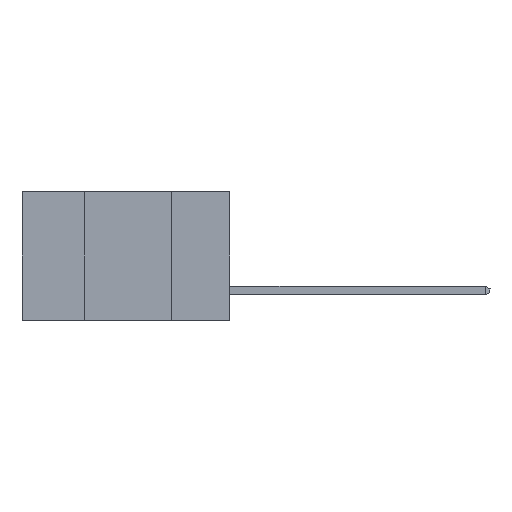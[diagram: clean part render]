
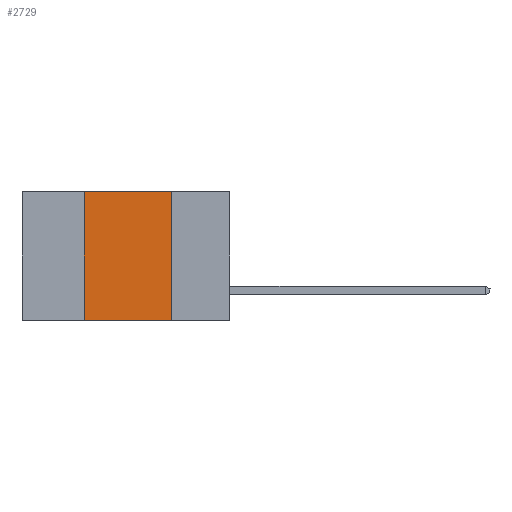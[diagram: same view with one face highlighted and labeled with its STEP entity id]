
A CAD part, left-side view. The second image highlights one B-rep face of the part: STEP entity #2729.
In plain terms, the highlighted planar face has unit normal (-1, 0, 0).
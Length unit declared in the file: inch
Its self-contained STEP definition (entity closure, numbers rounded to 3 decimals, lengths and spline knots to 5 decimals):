
#408 = ORIENTED_EDGE ( 'NONE', *, *, #13602, .F. ) ;
#1017 = EDGE_CURVE ( 'NONE', #12501, #17342, #10388, .T. ) ;
#1436 = VERTEX_POINT ( 'NONE', #19409 ) ;
#1492 = DIRECTION ( 'NONE',  ( 0., -1., 0. ) ) ;
#1813 = LINE ( 'NONE', #13632, #11678 ) ;
#1953 = CARTESIAN_POINT ( 'NONE',  ( 0., 0.17, -0.37 ) ) ;
#2729 = ADVANCED_FACE ( 'NONE', ( #10214 ), #8572, .F. ) ;
#2886 = DIRECTION ( 'NONE',  ( 0., 0., -1. ) ) ;
#4123 = AXIS2_PLACEMENT_3D ( 'NONE', #11872, #16969, #15203 ) ;
#4534 = CARTESIAN_POINT ( 'NONE',  ( 0., 0.17, -0.37 ) ) ;
#5583 = ORIENTED_EDGE ( 'NONE', *, *, #14785, .T. ) ;
#5584 = VERTEX_POINT ( 'NONE', #8233 ) ;
#6605 = LINE ( 'NONE', #11573, #21683 ) ;
#7022 = DIRECTION ( 'NONE',  ( 0., 0., 1. ) ) ;
#8233 = CARTESIAN_POINT ( 'NONE',  ( 0., 0.42, -0.37 ) ) ;
#8572 = PLANE ( 'NONE',  #4123 ) ;
#10214 = FACE_OUTER_BOUND ( 'NONE', #13310, .T. ) ;
#10388 = LINE ( 'NONE', #4534, #18707 ) ;
#10633 = ORIENTED_EDGE ( 'NONE', *, *, #1017, .F. ) ;
#11573 = CARTESIAN_POINT ( 'NONE',  ( 0., 0.6, 0. ) ) ;
#11678 = VECTOR ( 'NONE', #1492, 39.37008 ) ;
#11872 = CARTESIAN_POINT ( 'NONE',  ( 0., 0.6, 0. ) ) ;
#12501 = VERTEX_POINT ( 'NONE', #14524 ) ;
#12985 = VECTOR ( 'NONE', #7022, 39.37008 ) ;
#13310 = EDGE_LOOP ( 'NONE', ( #10633, #18561, #408, #5583 ) ) ;
#13602 = EDGE_CURVE ( 'NONE', #5584, #1436, #21688, .T. ) ;
#13632 = CARTESIAN_POINT ( 'NONE',  ( 0., 0.6, -0.37 ) ) ;
#14524 = CARTESIAN_POINT ( 'NONE',  ( 0., 0.17, 0. ) ) ;
#14785 = EDGE_CURVE ( 'NONE', #5584, #17342, #1813, .T. ) ;
#15203 = DIRECTION ( 'NONE',  ( 0., 0., -1. ) ) ;
#16969 = DIRECTION ( 'NONE',  ( 1., 0., 0. ) ) ;
#16988 = DIRECTION ( 'NONE',  ( 0., -1., 0. ) ) ;
#17342 = VERTEX_POINT ( 'NONE', #1953 ) ;
#18561 = ORIENTED_EDGE ( 'NONE', *, *, #20703, .F. ) ;
#18707 = VECTOR ( 'NONE', #2886, 39.37008 ) ;
#19409 = CARTESIAN_POINT ( 'NONE',  ( 0., 0.42, 0. ) ) ;
#20143 = CARTESIAN_POINT ( 'NONE',  ( 0., 0.42, -0.37 ) ) ;
#20703 = EDGE_CURVE ( 'NONE', #1436, #12501, #6605, .T. ) ;
#21683 = VECTOR ( 'NONE', #16988, 39.37008 ) ;
#21688 = LINE ( 'NONE', #20143, #12985 ) ;
